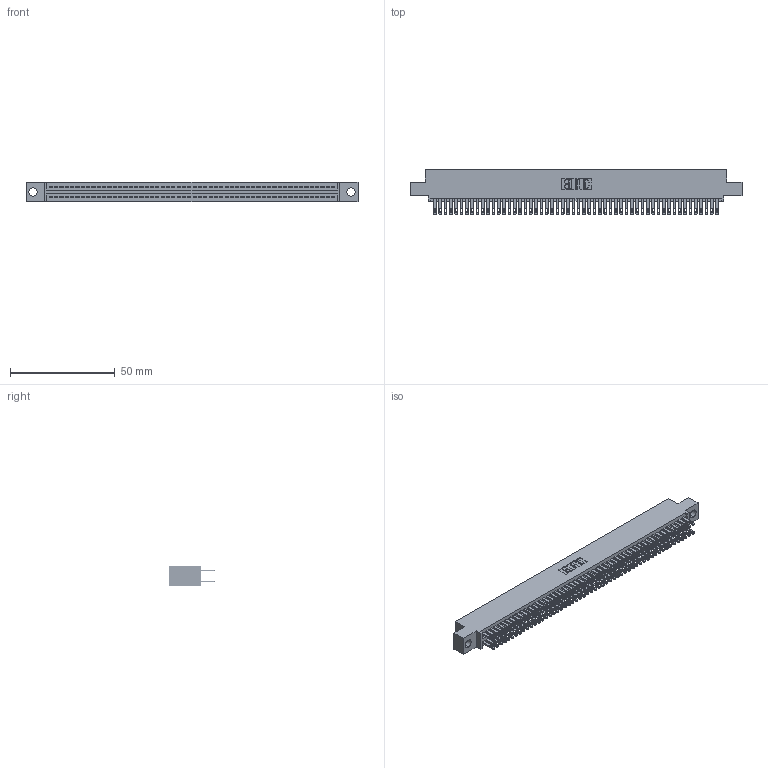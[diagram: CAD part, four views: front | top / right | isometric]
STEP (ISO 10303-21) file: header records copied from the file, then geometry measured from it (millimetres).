
FILE_DESCRIPTION (( 'STEP AP203' ), '1' );
FILE_NAME ('345-108-500-504.STEP', '2018-10-07T04:43:20', ( '' ), ( '' ), 'SwSTEP 2.0', 'SolidWorks 2016', '' );
FILE_SCHEMA (( 'CONFIG_CONTROL_DESIGN' ));
Length unit declared in the file: inch
Products named in the file (3): 345 Part_0.110 Offset - 0.156 Dia-TH; 345-292-001_345-293-100; 345-108-500-504
Assembly tree (109 placements, depth 2):
  345-108-500-504
    345 Part_0.110 Offset - 0.156 Dia-TH
    345-292-001_345-293-100  x108
Bounding box: 158.37 x 21.51 x 9.4 mm (x, y, z)
Volume: 15664.3 mm3; surface area: 24396.5 mm2
Topology: 109 solids, 109 shells, 5098 faces, 15581 edges, 10386 vertices
Faces by surface type: plane 3000, cylinder 2098
Entity records: 40819 total; most frequent: CARTESIAN_POINT 6832, ORIENTED_EDGE 6766, DIRECTION 6011, EDGE_CURVE 3383, VECTOR 3031, LINE 3031, VERTEX_POINT 2254, AXIS2_PLACEMENT_3D 1490
